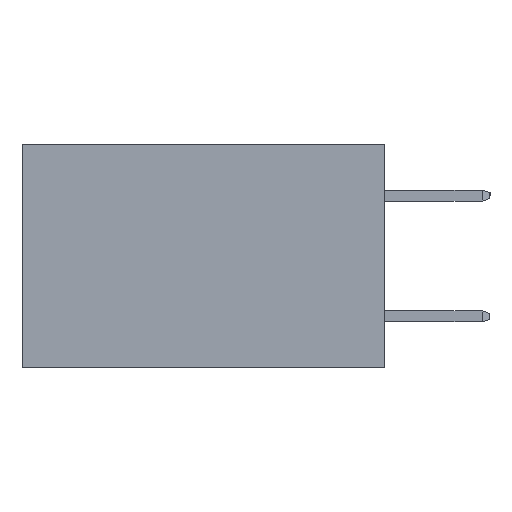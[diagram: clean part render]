
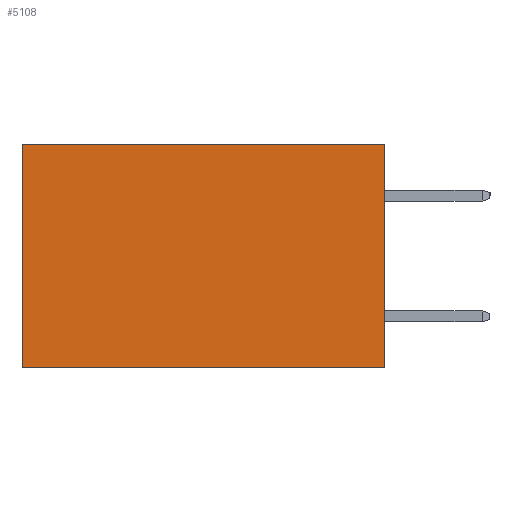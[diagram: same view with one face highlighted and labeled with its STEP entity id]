
A CAD part, left-side view. The second image highlights one B-rep face of the part: STEP entity #5108.
In plain terms, the highlighted planar face has unit normal (-1, 0, 0).
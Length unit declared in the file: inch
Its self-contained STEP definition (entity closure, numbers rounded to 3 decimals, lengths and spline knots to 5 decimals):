
#857 = ORIENTED_EDGE ( 'NONE', *, *, #4551, .T. ) ;
#864 = LINE ( 'NONE', #9203, #2893 ) ;
#886 = CARTESIAN_POINT ( 'NONE',  ( 0.2615, 0.6, -0.37 ) ) ;
#1053 = ORIENTED_EDGE ( 'NONE', *, *, #1605, .T. ) ;
#1250 = FACE_OUTER_BOUND ( 'NONE', #12950, .T. ) ;
#1317 = DIRECTION ( 'NONE',  ( 0., 0., -1. ) ) ;
#1605 = EDGE_CURVE ( 'NONE', #2967, #10677, #8415, .T. ) ;
#1626 = CARTESIAN_POINT ( 'NONE',  ( 0.2615, 0., -0.37 ) ) ;
#1916 = CARTESIAN_POINT ( 'NONE',  ( 0.2615, 0., 0. ) ) ;
#2424 = PLANE ( 'NONE',  #13439 ) ;
#2477 = DIRECTION ( 'NONE',  ( 0., 1., 0. ) ) ;
#2893 = VECTOR ( 'NONE', #5112, 39.37008 ) ;
#2967 = VERTEX_POINT ( 'NONE', #10384 ) ;
#3222 = DIRECTION ( 'NONE',  ( 0., 1., 0. ) ) ;
#3454 = DIRECTION ( 'NONE',  ( 0., 0., -1. ) ) ;
#3873 = ORIENTED_EDGE ( 'NONE', *, *, #11683, .F. ) ;
#4272 = CARTESIAN_POINT ( 'NONE',  ( 0.2615, 0., -0.37 ) ) ;
#4551 = EDGE_CURVE ( 'NONE', #10677, #11551, #864, .T. ) ;
#5053 = VECTOR ( 'NONE', #2477, 39.37008 ) ;
#5108 = ADVANCED_FACE ( 'NONE', ( #1250 ), #2424, .F. ) ;
#5112 = DIRECTION ( 'NONE',  ( 0., 0., -1. ) ) ;
#5237 = CARTESIAN_POINT ( 'NONE',  ( 0.2615, 0.6, 0. ) ) ;
#5267 = CARTESIAN_POINT ( 'NONE',  ( 0.2615, 0., -0.37 ) ) ;
#6257 = LINE ( 'NONE', #10409, #10957 ) ;
#6462 = EDGE_CURVE ( 'NONE', #2967, #9155, #6257, .T. ) ;
#8415 = LINE ( 'NONE', #1916, #11171 ) ;
#9155 = VERTEX_POINT ( 'NONE', #1626 ) ;
#9203 = CARTESIAN_POINT ( 'NONE',  ( 0.2615, 0.6, -0.37 ) ) ;
#9566 = ORIENTED_EDGE ( 'NONE', *, *, #6462, .F. ) ;
#10384 = CARTESIAN_POINT ( 'NONE',  ( 0.2615, 0., 0. ) ) ;
#10409 = CARTESIAN_POINT ( 'NONE',  ( 0.2615, 0., -0.37 ) ) ;
#10677 = VERTEX_POINT ( 'NONE', #5237 ) ;
#10957 = VECTOR ( 'NONE', #3454, 39.37008 ) ;
#11171 = VECTOR ( 'NONE', #3222, 39.37008 ) ;
#11551 = VERTEX_POINT ( 'NONE', #886 ) ;
#11683 = EDGE_CURVE ( 'NONE', #9155, #11551, #11814, .T. ) ;
#11769 = DIRECTION ( 'NONE',  ( 1., 0., 0. ) ) ;
#11814 = LINE ( 'NONE', #5267, #5053 ) ;
#12950 = EDGE_LOOP ( 'NONE', ( #857, #3873, #9566, #1053 ) ) ;
#13439 = AXIS2_PLACEMENT_3D ( 'NONE', #4272, #11769, #1317 ) ;
